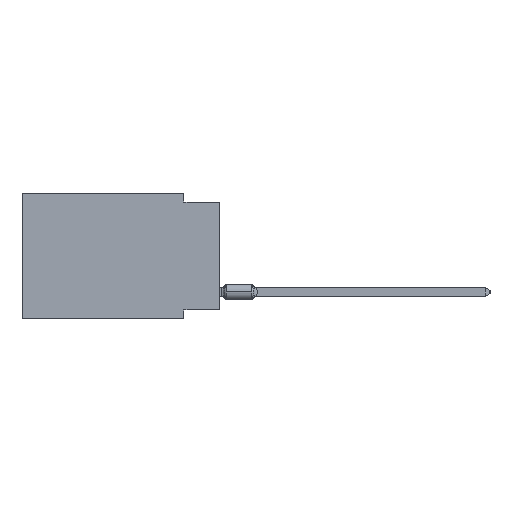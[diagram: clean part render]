
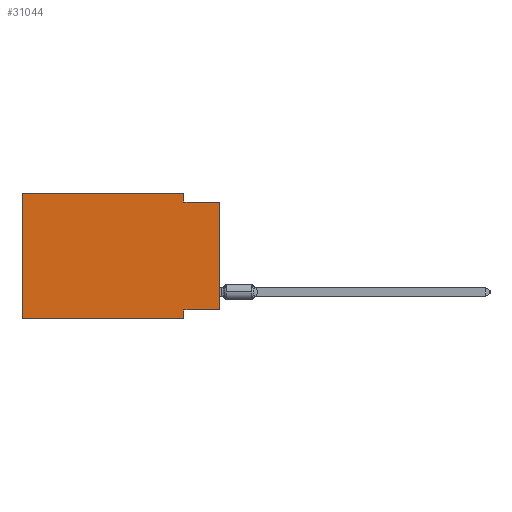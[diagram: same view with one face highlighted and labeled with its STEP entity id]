
A CAD part, left-side view. The second image highlights one B-rep face of the part: STEP entity #31044.
In plain terms, the highlighted planar face has unit normal (-1, 0, 0).
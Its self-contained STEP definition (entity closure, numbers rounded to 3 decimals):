
#912 = DIRECTION ( 'NONE',  ( 0., 0., 1. ) ) ;
#1333 = EDGE_CURVE ( 'NONE', #86038, #14812, #75604, .T. ) ;
#3463 = CARTESIAN_POINT ( 'NONE',  ( 0., 13.97, -8.89 ) ) ;
#3516 = VECTOR ( 'NONE', #71715, 1000. ) ;
#3908 = DIRECTION ( 'NONE',  ( 0., 0., -1. ) ) ;
#6197 = LINE ( 'NONE', #77844, #42461 ) ;
#13448 = VERTEX_POINT ( 'NONE', #100766 ) ;
#14812 = VERTEX_POINT ( 'NONE', #47215 ) ;
#15668 = DIRECTION ( 'NONE',  ( 0., 0., 1. ) ) ;
#18245 = VERTEX_POINT ( 'NONE', #102692 ) ;
#20264 = ORIENTED_EDGE ( 'NONE', *, *, #96443, .F. ) ;
#21960 = CARTESIAN_POINT ( 'NONE',  ( 0., 13.97, 0. ) ) ;
#22479 = DIRECTION ( 'NONE',  ( 0., -1., 0. ) ) ;
#27542 = ORIENTED_EDGE ( 'NONE', *, *, #65119, .T. ) ;
#30710 = VERTEX_POINT ( 'NONE', #74846 ) ;
#31044 = ADVANCED_FACE ( 'NONE', ( #46856 ), #78977, .F. ) ;
#34808 = ORIENTED_EDGE ( 'NONE', *, *, #65996, .F. ) ;
#35063 = DIRECTION ( 'NONE',  ( 0., -1., 0. ) ) ;
#37577 = CARTESIAN_POINT ( 'NONE',  ( 0., 2.54, 0. ) ) ;
#38276 = VECTOR ( 'NONE', #3908, 1000. ) ;
#39176 = LINE ( 'NONE', #94495, #71491 ) ;
#42461 = VECTOR ( 'NONE', #15668, 1000. ) ;
#46720 = CARTESIAN_POINT ( 'NONE',  ( 0., 13.97, -8.89 ) ) ;
#46734 = ORIENTED_EDGE ( 'NONE', *, *, #47216, .F. ) ;
#46856 = FACE_OUTER_BOUND ( 'NONE', #78154, .T. ) ;
#47216 = EDGE_CURVE ( 'NONE', #30710, #70247, #61986, .T. ) ;
#47215 = CARTESIAN_POINT ( 'NONE',  ( 0., 2.54, -8.89 ) ) ;
#47375 = CARTESIAN_POINT ( 'NONE',  ( 0., 13.97, 0. ) ) ;
#48560 = VECTOR ( 'NONE', #74323, 1000. ) ;
#49430 = ORIENTED_EDGE ( 'NONE', *, *, #85879, .F. ) ;
#49711 = ORIENTED_EDGE ( 'NONE', *, *, #58169, .F. ) ;
#50096 = CARTESIAN_POINT ( 'NONE',  ( 0., 0., -0.635 ) ) ;
#52443 = VECTOR ( 'NONE', #912, 1000. ) ;
#55092 = ORIENTED_EDGE ( 'NONE', *, *, #55152, .F. ) ;
#55152 = EDGE_CURVE ( 'NONE', #18245, #63824, #39176, .T. ) ;
#56564 = VECTOR ( 'NONE', #35063, 1000. ) ;
#58169 = EDGE_CURVE ( 'NONE', #70247, #85668, #59744, .T. ) ;
#58522 = LINE ( 'NONE', #50096, #48560 ) ;
#59744 = LINE ( 'NONE', #37577, #38276 ) ;
#61837 = DIRECTION ( 'NONE',  ( 0., 1., 0. ) ) ;
#61986 = LINE ( 'NONE', #21960, #91299 ) ;
#63824 = VERTEX_POINT ( 'NONE', #100924 ) ;
#65119 = EDGE_CURVE ( 'NONE', #18245, #13448, #83567, .T. ) ;
#65996 = EDGE_CURVE ( 'NONE', #86038, #30710, #6197, .T. ) ;
#69645 = LINE ( 'NONE', #78581, #3516 ) ;
#70247 = VERTEX_POINT ( 'NONE', #97698 ) ;
#71491 = VECTOR ( 'NONE', #61837, 1000. ) ;
#71715 = DIRECTION ( 'NONE',  ( 0., 0., -1. ) ) ;
#74323 = DIRECTION ( 'NONE',  ( 0., -1., 0. ) ) ;
#74846 = CARTESIAN_POINT ( 'NONE',  ( 0., 13.97, 0. ) ) ;
#74918 = AXIS2_PLACEMENT_3D ( 'NONE', #47375, #79494, #95827 ) ;
#75604 = LINE ( 'NONE', #3463, #56564 ) ;
#77844 = CARTESIAN_POINT ( 'NONE',  ( 0., 13.97, 0. ) ) ;
#78154 = EDGE_LOOP ( 'NONE', ( #27542, #49430, #49711, #46734, #34808, #97744, #20264, #55092 ) ) ;
#78581 = CARTESIAN_POINT ( 'NONE',  ( 0., 2.54, -8.89 ) ) ;
#78977 = PLANE ( 'NONE',  #74918 ) ;
#79494 = DIRECTION ( 'NONE',  ( 1., 0., 0. ) ) ;
#83049 = CARTESIAN_POINT ( 'NONE',  ( 0., 0., 0. ) ) ;
#83567 = LINE ( 'NONE', #83049, #52443 ) ;
#85668 = VERTEX_POINT ( 'NONE', #100742 ) ;
#85879 = EDGE_CURVE ( 'NONE', #85668, #13448, #58522, .T. ) ;
#86038 = VERTEX_POINT ( 'NONE', #46720 ) ;
#91299 = VECTOR ( 'NONE', #22479, 1000. ) ;
#94495 = CARTESIAN_POINT ( 'NONE',  ( 0., 0., -8.255 ) ) ;
#95827 = DIRECTION ( 'NONE',  ( 0., 0., -1. ) ) ;
#96443 = EDGE_CURVE ( 'NONE', #63824, #14812, #69645, .T. ) ;
#97698 = CARTESIAN_POINT ( 'NONE',  ( 0., 2.54, 0. ) ) ;
#97744 = ORIENTED_EDGE ( 'NONE', *, *, #1333, .T. ) ;
#100742 = CARTESIAN_POINT ( 'NONE',  ( 0., 2.54, -0.635 ) ) ;
#100766 = CARTESIAN_POINT ( 'NONE',  ( 0., 0., -0.635 ) ) ;
#100924 = CARTESIAN_POINT ( 'NONE',  ( 0., 2.54, -8.255 ) ) ;
#102692 = CARTESIAN_POINT ( 'NONE',  ( 0., 0., -8.255 ) ) ;
